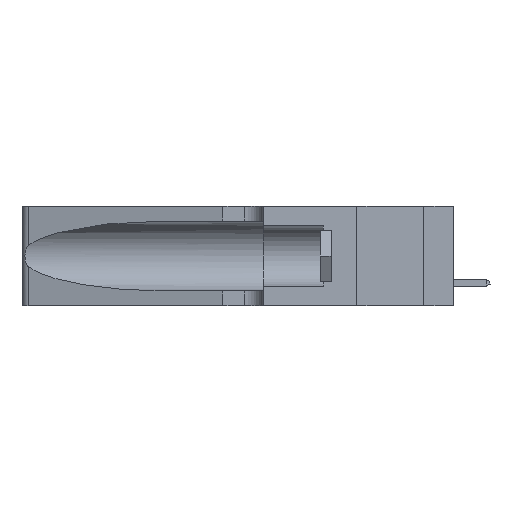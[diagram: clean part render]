
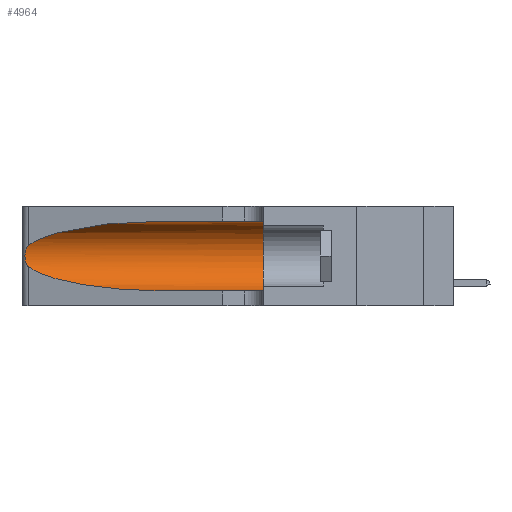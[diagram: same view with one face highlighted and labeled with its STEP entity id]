
A CAD part, left-side view. The second image highlights one B-rep face of the part: STEP entity #4964.
In plain terms, the highlighted cylindrical face has radius 3.308 mm (diameter 6.617 mm), a partial arc.
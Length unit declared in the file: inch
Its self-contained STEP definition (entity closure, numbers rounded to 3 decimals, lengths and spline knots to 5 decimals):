
#822 = EDGE_CURVE ( 'NONE', #16689, #20341, #15801, .T. ) ;
#1841 = CARTESIAN_POINT ( 'NONE',  ( 0.2373, 1.15595, 0.28018 ) ) ;
#1901 = CARTESIAN_POINT ( 'NONE',  ( 0.1305, 0.72297, 0.05475 ) ) ;
#2143 = CARTESIAN_POINT ( 'NONE',  ( 0.25639, 1.23184, 0.21858 ) ) ;
#2328 = CARTESIAN_POINT ( 'NONE',  ( 0.18966, 0.96281, 0.05475 ) ) ;
#3490 = AXIS2_PLACEMENT_3D ( 'NONE', #16779, #4436, #18889 ) ;
#3550 = ORIENTED_EDGE ( 'NONE', *, *, #11046, .T. ) ;
#3633 = LINE ( 'NONE', #5756, #17030 ) ;
#4436 = DIRECTION ( 'NONE',  ( 0., 1., 0. ) ) ;
#4597 = CARTESIAN_POINT ( 'NONE',  ( 0.26018, 1.23835, 0.19895 ) ) ;
#4886 = EDGE_CURVE ( 'NONE', #20341, #25893, #21312, .T. ) ;
#4964 = ADVANCED_FACE ( 'NONE', ( #16935 ), #12059, .F. ) ;
#5756 = CARTESIAN_POINT ( 'NONE',  ( 0.1305, 1.61858, 0.31525 ) ) ;
#6072 = CIRCLE ( 'NONE', #3490, 0.13025 ) ;
#6414 = VERTEX_POINT ( 'NONE', #22600 ) ;
#6613 = CARTESIAN_POINT ( 'NONE',  ( 0.25555, 1.22994, 0.2215 ) ) ;
#6650 = VECTOR ( 'NONE', #20761, 39.37008 ) ;
#6980 = CARTESIAN_POINT ( 'NONE',  ( 0.25639, 1.23186, 0.15144 ) ) ;
#7081 = EDGE_CURVE ( 'NONE', #6414, #23086, #6072, .T. ) ;
#8539 = CARTESIAN_POINT ( 'NONE',  ( 0.25487, 1.22718, 0.14631 ) ) ;
#9284 = LINE ( 'NONE', #20493, #6650 ) ;
#10455 = CARTESIAN_POINT ( 'NONE',  ( 0.26075, 1.23896, 0.19203 ) ) ;
#10620 =( BOUNDED_CURVE ( )  B_SPLINE_CURVE ( 3, ( #8539, #12728, #2328, #19055 ),
 .UNSPECIFIED., .F., .F. ) 
 B_SPLINE_CURVE_WITH_KNOTS ( ( 4, 4 ),
 ( 3.44316, 4.71239 ),
 .UNSPECIFIED. ) 
 CURVE ( )  GEOMETRIC_REPRESENTATION_ITEM ( )  RATIONAL_B_SPLINE_CURVE ( ( 1., 0.87, 0.87, 1. ) ) 
 REPRESENTATION_ITEM ( '' )  );
#10626 = CARTESIAN_POINT ( 'NONE',  ( 0.25789, 1.23486, 0.15765 ) ) ;
#11046 = EDGE_CURVE ( 'NONE', #15484, #23086, #9284, .T. ) ;
#11343 = AXIS2_PLACEMENT_3D ( 'NONE', #24395, #16157, #24489 ) ;
#12059 = CYLINDRICAL_SURFACE ( 'NONE', #11343, 0.13025 ) ;
#12728 = CARTESIAN_POINT ( 'NONE',  ( 0.2373, 1.15595, 0.08982 ) ) ;
#14171 = DIRECTION ( 'NONE',  ( 0., -1., 0. ) ) ;
#14746 = CARTESIAN_POINT ( 'NONE',  ( 0.25856, 1.23593, 0.16098 ) ) ;
#15104 = CARTESIAN_POINT ( 'NONE',  ( 0.1305, 0.72297, 0.31525 ) ) ;
#15484 = VERTEX_POINT ( 'NONE', #1901 ) ;
#15582 = ORIENTED_EDGE ( 'NONE', *, *, #4886, .T. ) ;
#15801 =( BOUNDED_CURVE ( )  B_SPLINE_CURVE ( 3, ( #16378, #26906, #1841, #16469 ),
 .UNSPECIFIED., .F., .F. ) 
 B_SPLINE_CURVE_WITH_KNOTS ( ( 4, 4 ),
 ( 1.5708, 2.84003 ),
 .UNSPECIFIED. ) 
 CURVE ( )  GEOMETRIC_REPRESENTATION_ITEM ( )  RATIONAL_B_SPLINE_CURVE ( ( 1., 0.87, 0.87, 1. ) ) 
 REPRESENTATION_ITEM ( '' )  );
#16157 = DIRECTION ( 'NONE',  ( 0., -1., 0. ) ) ;
#16378 = CARTESIAN_POINT ( 'NONE',  ( 0.1305, 0.72297, 0.31525 ) ) ;
#16469 = CARTESIAN_POINT ( 'NONE',  ( 0.25487, 1.22718, 0.22369 ) ) ;
#16689 = VERTEX_POINT ( 'NONE', #15104 ) ;
#16779 = CARTESIAN_POINT ( 'NONE',  ( 0.1305, 0.35, 0.185 ) ) ;
#16862 = ORIENTED_EDGE ( 'NONE', *, *, #21182, .T. ) ;
#16912 = CARTESIAN_POINT ( 'NONE',  ( 0.25787, 1.23484, 0.2124 ) ) ;
#16935 = FACE_OUTER_BOUND ( 'NONE', #22193, .T. ) ;
#17030 = VECTOR ( 'NONE', #14171, 39.37008 ) ;
#17599 = CARTESIAN_POINT ( 'NONE',  ( 0.1305, 0.35, 0.05475 ) ) ;
#18889 = DIRECTION ( 'NONE',  ( 0., 0., 1. ) ) ;
#18948 = CARTESIAN_POINT ( 'NONE',  ( 0.25487, 1.22718, 0.22369 ) ) ;
#19055 = CARTESIAN_POINT ( 'NONE',  ( 0.1305, 0.72297, 0.05475 ) ) ;
#19939 = ORIENTED_EDGE ( 'NONE', *, *, #7081, .F. ) ;
#20341 = VERTEX_POINT ( 'NONE', #24365 ) ;
#20493 = CARTESIAN_POINT ( 'NONE',  ( 0.1305, 1.61858, 0.05475 ) ) ;
#20761 = DIRECTION ( 'NONE',  ( 0., -1., 0. ) ) ;
#20858 = CARTESIAN_POINT ( 'NONE',  ( 0.25555, 1.22993, 0.14849 ) ) ;
#20949 = CARTESIAN_POINT ( 'NONE',  ( 0.25487, 1.22718, 0.14631 ) ) ;
#21017 = EDGE_CURVE ( 'NONE', #16689, #6414, #3633, .T. ) ;
#21049 = CARTESIAN_POINT ( 'NONE',  ( 0.25854, 1.2359, 0.20912 ) ) ;
#21182 = EDGE_CURVE ( 'NONE', #25893, #15484, #10620, .T. ) ;
#21312 = B_SPLINE_CURVE_WITH_KNOTS ( 'NONE', 3,
 ( #18948, #6613, #2143, #16912, #21049, #4597, #10455, #23028, #23122, #14746, #10626, #6980, #20858, #20949 ),
 .UNSPECIFIED., .F., .F.,
 ( 4, 2, 2, 2, 2, 2, 4 ),
 ( 0., 0.00027, 0.00053, 0.00107, 0.0016, 0.00187, 0.00214 ),
 .UNSPECIFIED. ) ;
#22193 = EDGE_LOOP ( 'NONE', ( #24581, #15582, #16862, #3550, #19939, #25793 ) ) ;
#22600 = CARTESIAN_POINT ( 'NONE',  ( 0.1305, 0.35, 0.31525 ) ) ;
#23028 = CARTESIAN_POINT ( 'NONE',  ( 0.26075, 1.23896, 0.178 ) ) ;
#23086 = VERTEX_POINT ( 'NONE', #17599 ) ;
#23122 = CARTESIAN_POINT ( 'NONE',  ( 0.26017, 1.23833, 0.17102 ) ) ;
#24365 = CARTESIAN_POINT ( 'NONE',  ( 0.25487, 1.22718, 0.22369 ) ) ;
#24395 = CARTESIAN_POINT ( 'NONE',  ( 0.1305, 1.61858, 0.185 ) ) ;
#24489 = DIRECTION ( 'NONE',  ( 0., 0., -1. ) ) ;
#24581 = ORIENTED_EDGE ( 'NONE', *, *, #822, .T. ) ;
#25793 = ORIENTED_EDGE ( 'NONE', *, *, #21017, .F. ) ;
#25893 = VERTEX_POINT ( 'NONE', #26495 ) ;
#26495 = CARTESIAN_POINT ( 'NONE',  ( 0.25487, 1.22718, 0.14631 ) ) ;
#26906 = CARTESIAN_POINT ( 'NONE',  ( 0.18966, 0.96281, 0.31525 ) ) ;
